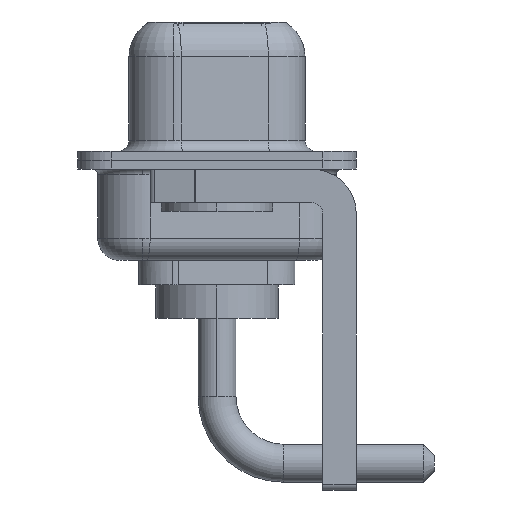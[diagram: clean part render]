
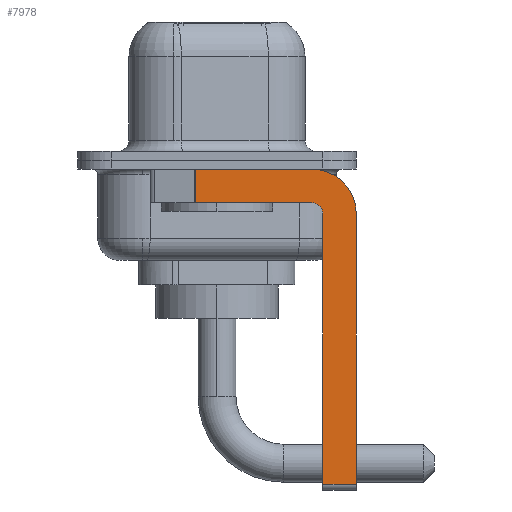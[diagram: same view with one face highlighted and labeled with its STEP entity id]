
A CAD part, left-side view. The second image highlights one B-rep face of the part: STEP entity #7978.
In plain terms, the highlighted planar face has unit normal (-1, 0, 0).
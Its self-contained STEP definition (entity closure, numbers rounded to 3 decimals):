
#629 = CARTESIAN_POINT ( 'NONE',  ( -2.9, -6.25, -2.4 ) ) ;
#943 = CARTESIAN_POINT ( 'NONE',  ( -2.9, 3., -0.4 ) ) ;
#1188 = CARTESIAN_POINT ( 'NONE',  ( -2.9, -4.75, -14.8 ) ) ;
#1368 = VECTOR ( 'NONE', #5238, 1000. ) ;
#1740 = CARTESIAN_POINT ( 'NONE',  ( -2.9, 0.978, -0.4 ) ) ;
#1794 = EDGE_CURVE ( 'NONE', #4404, #4366, #9252, .T. ) ;
#1831 = DIRECTION ( 'NONE',  ( 0., 0., -1. ) ) ;
#1898 = DIRECTION ( 'NONE',  ( -1., 0., 0. ) ) ;
#1950 = VERTEX_POINT ( 'NONE', #5156 ) ;
#2482 = CARTESIAN_POINT ( 'NONE',  ( -2.9, -4.25, -0.4 ) ) ;
#2873 = CARTESIAN_POINT ( 'NONE',  ( -2.9, 0.978, -1.9 ) ) ;
#2898 = CARTESIAN_POINT ( 'NONE',  ( -2.9, -4.25, -2.4 ) ) ;
#3038 = VECTOR ( 'NONE', #13002, 1000. ) ;
#3122 = AXIS2_PLACEMENT_3D ( 'NONE', #7792, #8842, #3824 ) ;
#3152 = VERTEX_POINT ( 'NONE', #12891 ) ;
#3294 = VECTOR ( 'NONE', #3344, 1000. ) ;
#3344 = DIRECTION ( 'NONE',  ( 0., 1., 0. ) ) ;
#3628 = VECTOR ( 'NONE', #8239, 1000. ) ;
#3671 = ORIENTED_EDGE ( 'NONE', *, *, #11352, .F. ) ;
#3718 = ORIENTED_EDGE ( 'NONE', *, *, #10118, .F. ) ;
#3824 = DIRECTION ( 'NONE',  ( 0., 0., -1. ) ) ;
#4160 = DIRECTION ( 'NONE',  ( 1., 0., 0. ) ) ;
#4366 = VERTEX_POINT ( 'NONE', #11153 ) ;
#4404 = VERTEX_POINT ( 'NONE', #2482 ) ;
#4462 = VERTEX_POINT ( 'NONE', #5531 ) ;
#4574 = AXIS2_PLACEMENT_3D ( 'NONE', #2898, #1898, #5101 ) ;
#4678 = EDGE_CURVE ( 'NONE', #1950, #3152, #12259, .T. ) ;
#5003 = VERTEX_POINT ( 'NONE', #5762 ) ;
#5010 = ORIENTED_EDGE ( 'NONE', *, *, #7859, .T. ) ;
#5101 = DIRECTION ( 'NONE',  ( 0., 0., 1. ) ) ;
#5156 = CARTESIAN_POINT ( 'NONE',  ( -2.9, -4.75, -14.55 ) ) ;
#5238 = DIRECTION ( 'NONE',  ( 0., 0., 1. ) ) ;
#5265 = CARTESIAN_POINT ( 'NONE',  ( -2.9, -4.25, -14.55 ) ) ;
#5531 = CARTESIAN_POINT ( 'NONE',  ( -2.9, 0.978, -1.9 ) ) ;
#5762 = CARTESIAN_POINT ( 'NONE',  ( -2.9, -4.75, -2.4 ) ) ;
#5923 = LINE ( 'NONE', #943, #3038 ) ;
#5936 = DIRECTION ( 'NONE',  ( 0., 0., -1. ) ) ;
#6006 = PLANE ( 'NONE',  #8957 ) ;
#6074 = ORIENTED_EDGE ( 'NONE', *, *, #4678, .T. ) ;
#6285 = VECTOR ( 'NONE', #1831, 1000. ) ;
#6449 = VECTOR ( 'NONE', #5936, 1000. ) ;
#7133 = CARTESIAN_POINT ( 'NONE',  ( -2.9, -4.25, -2.4 ) ) ;
#7188 = LINE ( 'NONE', #12272, #3294 ) ;
#7389 = EDGE_CURVE ( 'NONE', #7862, #4404, #5923, .T. ) ;
#7792 = CARTESIAN_POINT ( 'NONE',  ( -2.9, -4.25, -2.4 ) ) ;
#7859 = EDGE_CURVE ( 'NONE', #7862, #4462, #10813, .T. ) ;
#7862 = VERTEX_POINT ( 'NONE', #1740 ) ;
#7978 = ADVANCED_FACE ( 'NONE', ( #11287 ), #6006, .F. ) ;
#8239 = DIRECTION ( 'NONE',  ( 0., -1., 0. ) ) ;
#8586 = CIRCLE ( 'NONE', #4574, 0.5 ) ;
#8842 = DIRECTION ( 'NONE',  ( 1., 0., 0. ) ) ;
#8865 = EDGE_LOOP ( 'NONE', ( #10133, #5010, #10461, #3671, #3718, #6074, #10085, #9100 ) ) ;
#8957 = AXIS2_PLACEMENT_3D ( 'NONE', #7133, #4160, #10222 ) ;
#9100 = ORIENTED_EDGE ( 'NONE', *, *, #1794, .F. ) ;
#9252 = CIRCLE ( 'NONE', #3122, 2. ) ;
#9698 = CARTESIAN_POINT ( 'NONE',  ( -2.9, -4.25, -1.9 ) ) ;
#10085 = ORIENTED_EDGE ( 'NONE', *, *, #11995, .F. ) ;
#10118 = EDGE_CURVE ( 'NONE', #1950, #5003, #10246, .T. ) ;
#10133 = ORIENTED_EDGE ( 'NONE', *, *, #7389, .F. ) ;
#10222 = DIRECTION ( 'NONE',  ( 0., 0., -1. ) ) ;
#10246 = LINE ( 'NONE', #1188, #1368 ) ;
#10461 = ORIENTED_EDGE ( 'NONE', *, *, #11065, .F. ) ;
#10813 = LINE ( 'NONE', #2873, #6449 ) ;
#11065 = EDGE_CURVE ( 'NONE', #11992, #4462, #7188, .T. ) ;
#11153 = CARTESIAN_POINT ( 'NONE',  ( -2.9, -6.25, -2.4 ) ) ;
#11287 = FACE_OUTER_BOUND ( 'NONE', #8865, .T. ) ;
#11352 = EDGE_CURVE ( 'NONE', #5003, #11992, #8586, .T. ) ;
#11761 = LINE ( 'NONE', #629, #6285 ) ;
#11992 = VERTEX_POINT ( 'NONE', #9698 ) ;
#11995 = EDGE_CURVE ( 'NONE', #4366, #3152, #11761, .T. ) ;
#12259 = LINE ( 'NONE', #5265, #3628 ) ;
#12272 = CARTESIAN_POINT ( 'NONE',  ( -2.9, -4.25, -1.9 ) ) ;
#12891 = CARTESIAN_POINT ( 'NONE',  ( -2.9, -6.25, -14.55 ) ) ;
#13002 = DIRECTION ( 'NONE',  ( 0., -1., 0. ) ) ;
